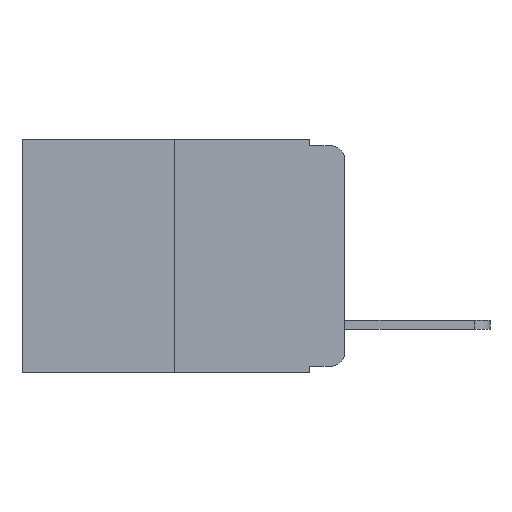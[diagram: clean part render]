
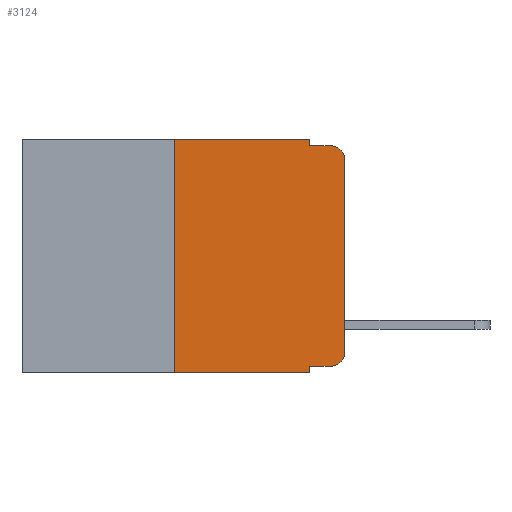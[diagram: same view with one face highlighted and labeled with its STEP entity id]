
A CAD part, left-side view. The second image highlights one B-rep face of the part: STEP entity #3124.
In plain terms, the highlighted planar face has unit normal (-1, 0, 0).
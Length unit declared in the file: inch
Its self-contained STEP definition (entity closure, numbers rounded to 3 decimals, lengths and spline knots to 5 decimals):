
#53 = DIRECTION ( 'NONE',  ( 0., -1., 0. ) ) ;
#63 = FACE_OUTER_BOUND ( 'NONE', #8875, .T. ) ;
#114 = VERTEX_POINT ( 'NONE', #3335 ) ;
#219 = CIRCLE ( 'NONE', #5521, 0.02 ) ;
#358 = ORIENTED_EDGE ( 'NONE', *, *, #4539, .T. ) ;
#361 = ORIENTED_EDGE ( 'NONE', *, *, #4540, .T. ) ;
#450 = ORIENTED_EDGE ( 'NONE', *, *, #4657, .F. ) ;
#651 = ORIENTED_EDGE ( 'NONE', *, *, #4959, .F. ) ;
#670 = ORIENTED_EDGE ( 'NONE', *, *, #7608, .F. ) ;
#787 = ORIENTED_EDGE ( 'NONE', *, *, #5025, .F. ) ;
#863 = VECTOR ( 'NONE', #2413, 39.37008 ) ;
#911 = ORIENTED_EDGE ( 'NONE', *, *, #3904, .T. ) ;
#1026 = ORIENTED_EDGE ( 'NONE', *, *, #5120, .T. ) ;
#1048 = ORIENTED_EDGE ( 'NONE', *, *, #5073, .T. ) ;
#1089 = LINE ( 'NONE', #9340, #6302 ) ;
#1369 = VERTEX_POINT ( 'NONE', #9040 ) ;
#1679 = VERTEX_POINT ( 'NONE', #12290 ) ;
#1834 = ORIENTED_EDGE ( 'NONE', *, *, #4603, .F. ) ;
#2058 = CARTESIAN_POINT ( 'NONE',  ( 0., 0.02, -0.313 ) ) ;
#2131 = LINE ( 'NONE', #8944, #9574 ) ;
#2324 = DIRECTION ( 'NONE',  ( 0., -1., 0. ) ) ;
#2354 = DIRECTION ( 'NONE',  ( 0., -1., 0. ) ) ;
#2413 = DIRECTION ( 'NONE',  ( 0., 0., -1. ) ) ;
#2460 = CARTESIAN_POINT ( 'NONE',  ( 0., 0.473, -0.343 ) ) ;
#2495 = LINE ( 'NONE', #4590, #5097 ) ;
#2605 = CARTESIAN_POINT ( 'NONE',  ( 0., 0.25, 0. ) ) ;
#3124 = ADVANCED_FACE ( 'NONE', ( #63 ), #7731, .F. ) ;
#3335 = CARTESIAN_POINT ( 'NONE',  ( 0., 0.051, -0.343 ) ) ;
#3639 = VERTEX_POINT ( 'NONE', #10671 ) ;
#3708 = LINE ( 'NONE', #6665, #8455 ) ;
#3904 = EDGE_CURVE ( 'NONE', #5194, #114, #7960, .T. ) ;
#4070 = DIRECTION ( 'NONE',  ( 1., 0., 0. ) ) ;
#4203 = DIRECTION ( 'NONE',  ( 0., 0., 1. ) ) ;
#4539 = EDGE_CURVE ( 'NONE', #7855, #1679, #2495, .T. ) ;
#4540 = EDGE_CURVE ( 'NONE', #1679, #3639, #7550, .T. ) ;
#4590 = CARTESIAN_POINT ( 'NONE',  ( 0., 0., 0. ) ) ;
#4602 = DIRECTION ( 'NONE',  ( 0., 0., -1. ) ) ;
#4603 = EDGE_CURVE ( 'NONE', #1369, #3639, #2131, .T. ) ;
#4657 = EDGE_CURVE ( 'NONE', #8656, #1369, #9097, .T. ) ;
#4764 = VERTEX_POINT ( 'NONE', #2605 ) ;
#4959 = EDGE_CURVE ( 'NONE', #5194, #4764, #11719, .T. ) ;
#5025 = EDGE_CURVE ( 'NONE', #7174, #114, #6824, .T. ) ;
#5073 = EDGE_CURVE ( 'NONE', #7174, #10610, #1089, .T. ) ;
#5097 = VECTOR ( 'NONE', #5418, 39.37008 ) ;
#5120 = EDGE_CURVE ( 'NONE', #10610, #7855, #219, .T. ) ;
#5194 = VERTEX_POINT ( 'NONE', #10828 ) ;
#5383 = CARTESIAN_POINT ( 'NONE',  ( 0., 0.02, -0.03 ) ) ;
#5418 = DIRECTION ( 'NONE',  ( 0., 0., 1. ) ) ;
#5521 = AXIS2_PLACEMENT_3D ( 'NONE', #2058, #8137, #8122 ) ;
#5580 = VECTOR ( 'NONE', #53, 39.37008 ) ;
#5710 = CARTESIAN_POINT ( 'NONE',  ( 0., 0.25, 0. ) ) ;
#5810 = DIRECTION ( 'NONE',  ( 0., 0., -1. ) ) ;
#6221 = DIRECTION ( 'NONE',  ( -1., 0., 0. ) ) ;
#6302 = VECTOR ( 'NONE', #2324, 39.37008 ) ;
#6436 = DIRECTION ( 'NONE',  ( 0., 0., -1. ) ) ;
#6665 = CARTESIAN_POINT ( 'NONE',  ( 0., 0.473, 0. ) ) ;
#6824 = LINE ( 'NONE', #11740, #7091 ) ;
#6874 = CARTESIAN_POINT ( 'NONE',  ( 0., 0.051, -0.333 ) ) ;
#7091 = VECTOR ( 'NONE', #6436, 39.37008 ) ;
#7174 = VERTEX_POINT ( 'NONE', #6874 ) ;
#7301 = CARTESIAN_POINT ( 'NONE',  ( 0., 0.02, -0.333 ) ) ;
#7550 = CIRCLE ( 'NONE', #9877, 0.02 ) ;
#7608 = EDGE_CURVE ( 'NONE', #4764, #8656, #3708, .T. ) ;
#7709 = CARTESIAN_POINT ( 'NONE',  ( 0., 0.473, 0. ) ) ;
#7730 = CARTESIAN_POINT ( 'NONE',  ( 0., 0.051, 0. ) ) ;
#7731 = PLANE ( 'NONE',  #11852 ) ;
#7855 = VERTEX_POINT ( 'NONE', #11193 ) ;
#7960 = LINE ( 'NONE', #2460, #5580 ) ;
#8122 = DIRECTION ( 'NONE',  ( 0., 0., -1. ) ) ;
#8137 = DIRECTION ( 'NONE',  ( -1., 0., 0. ) ) ;
#8455 = VECTOR ( 'NONE', #9623, 39.37008 ) ;
#8656 = VERTEX_POINT ( 'NONE', #7730 ) ;
#8875 = EDGE_LOOP ( 'NONE', ( #358, #361, #1834, #450, #670, #651, #911, #787, #1048, #1026 ) ) ;
#8944 = CARTESIAN_POINT ( 'NONE',  ( 0., 0.051, -0.01 ) ) ;
#9040 = CARTESIAN_POINT ( 'NONE',  ( 0., 0.051, -0.01 ) ) ;
#9097 = LINE ( 'NONE', #10626, #863 ) ;
#9340 = CARTESIAN_POINT ( 'NONE',  ( 0., 0.051, -0.333 ) ) ;
#9574 = VECTOR ( 'NONE', #2354, 39.37008 ) ;
#9623 = DIRECTION ( 'NONE',  ( 0., -1., 0. ) ) ;
#9685 = VECTOR ( 'NONE', #4203, 39.37008 ) ;
#9877 = AXIS2_PLACEMENT_3D ( 'NONE', #5383, #6221, #5810 ) ;
#10610 = VERTEX_POINT ( 'NONE', #7301 ) ;
#10626 = CARTESIAN_POINT ( 'NONE',  ( 0., 0.051, 0. ) ) ;
#10671 = CARTESIAN_POINT ( 'NONE',  ( 0., 0.02, -0.01 ) ) ;
#10828 = CARTESIAN_POINT ( 'NONE',  ( 0., 0.25, -0.343 ) ) ;
#11193 = CARTESIAN_POINT ( 'NONE',  ( 0., 0., -0.313 ) ) ;
#11719 = LINE ( 'NONE', #5710, #9685 ) ;
#11740 = CARTESIAN_POINT ( 'NONE',  ( 0., 0.051, 0. ) ) ;
#11852 = AXIS2_PLACEMENT_3D ( 'NONE', #7709, #4070, #4602 ) ;
#12290 = CARTESIAN_POINT ( 'NONE',  ( 0., 0., -0.03 ) ) ;
